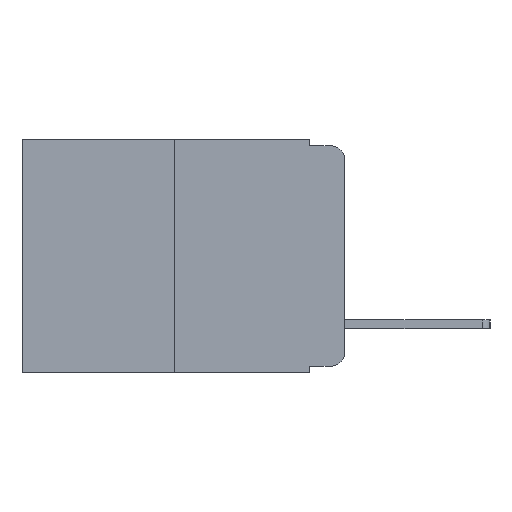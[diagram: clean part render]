
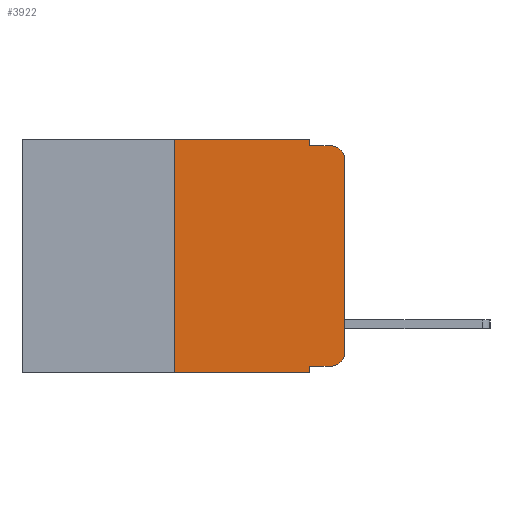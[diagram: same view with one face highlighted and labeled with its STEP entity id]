
A CAD part, left-side view. The second image highlights one B-rep face of the part: STEP entity #3922.
In plain terms, the highlighted planar face has unit normal (-1, 0, 0).
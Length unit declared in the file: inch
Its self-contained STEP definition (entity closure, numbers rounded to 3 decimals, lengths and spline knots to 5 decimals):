
#48 = PLANE ( 'NONE',  #1710 ) ;
#73 = DIRECTION ( 'NONE',  ( 0., 0., -1. ) ) ;
#90 = DIRECTION ( 'NONE',  ( 1., 0., 0. ) ) ;
#201 = DIRECTION ( 'NONE',  ( 0., 0., 1. ) ) ;
#320 = VERTEX_POINT ( 'NONE', #8663 ) ;
#596 = DIRECTION ( 'NONE',  ( 0., 0., -1. ) ) ;
#610 = VECTOR ( 'NONE', #3336, 39.37008 ) ;
#763 = EDGE_CURVE ( 'NONE', #1089, #12890, #6346, .T. ) ;
#775 = AXIS2_PLACEMENT_3D ( 'NONE', #8355, #8340, #7607 ) ;
#857 = CARTESIAN_POINT ( 'NONE',  ( 0., 0.25, 0. ) ) ;
#897 = CARTESIAN_POINT ( 'NONE',  ( 0., 0.25, 0. ) ) ;
#1089 = VERTEX_POINT ( 'NONE', #10288 ) ;
#1657 = EDGE_CURVE ( 'NONE', #2693, #8199, #9478, .T. ) ;
#1710 = AXIS2_PLACEMENT_3D ( 'NONE', #6113, #90, #73 ) ;
#2004 = ORIENTED_EDGE ( 'NONE', *, *, #11874, .T. ) ;
#2117 = CARTESIAN_POINT ( 'NONE',  ( 0., 0.051, 0. ) ) ;
#2319 = CARTESIAN_POINT ( 'NONE',  ( 0., 0., 0. ) ) ;
#2333 = ORIENTED_EDGE ( 'NONE', *, *, #3789, .T. ) ;
#2411 = CARTESIAN_POINT ( 'NONE',  ( 0., 0.051, -0.01 ) ) ;
#2581 = CARTESIAN_POINT ( 'NONE',  ( 0., 0.473, 0. ) ) ;
#2693 = VERTEX_POINT ( 'NONE', #897 ) ;
#2996 = VERTEX_POINT ( 'NONE', #2411 ) ;
#3309 = ORIENTED_EDGE ( 'NONE', *, *, #3371, .T. ) ;
#3336 = DIRECTION ( 'NONE',  ( 0., 0., -1. ) ) ;
#3371 = EDGE_CURVE ( 'NONE', #9353, #320, #12483, .T. ) ;
#3393 = LINE ( 'NONE', #2319, #8781 ) ;
#3564 = DIRECTION ( 'NONE',  ( 0., -1., 0. ) ) ;
#3789 = EDGE_CURVE ( 'NONE', #12726, #10171, #4030, .T. ) ;
#3831 = DIRECTION ( 'NONE',  ( 0., -1., 0. ) ) ;
#3922 = ADVANCED_FACE ( 'NONE', ( #8435 ), #48, .F. ) ;
#4030 = CIRCLE ( 'NONE', #6306, 0.02 ) ;
#4320 = ORIENTED_EDGE ( 'NONE', *, *, #12712, .F. ) ;
#4924 = CARTESIAN_POINT ( 'NONE',  ( 0., 0., -0.03 ) ) ;
#4969 = VECTOR ( 'NONE', #10505, 39.37008 ) ;
#4999 = VERTEX_POINT ( 'NONE', #11763 ) ;
#5079 = VECTOR ( 'NONE', #3831, 39.37008 ) ;
#5171 = VECTOR ( 'NONE', #9174, 39.37008 ) ;
#5239 = EDGE_CURVE ( 'NONE', #4999, #12890, #10244, .T. ) ;
#5328 = CARTESIAN_POINT ( 'NONE',  ( 0., 0.051, -0.343 ) ) ;
#5497 = LINE ( 'NONE', #8148, #5171 ) ;
#5764 = VECTOR ( 'NONE', #596, 39.37008 ) ;
#5983 = CARTESIAN_POINT ( 'NONE',  ( 0., 0.051, 0. ) ) ;
#6113 = CARTESIAN_POINT ( 'NONE',  ( 0., 0.473, 0. ) ) ;
#6256 = CARTESIAN_POINT ( 'NONE',  ( 0., 0.02, -0.01 ) ) ;
#6306 = AXIS2_PLACEMENT_3D ( 'NONE', #8937, #8924, #8656 ) ;
#6346 = LINE ( 'NONE', #2117, #610 ) ;
#6384 = ORIENTED_EDGE ( 'NONE', *, *, #5239, .T. ) ;
#6559 = EDGE_LOOP ( 'NONE', ( #2004, #2333, #11455, #4320, #10643, #8547, #6384, #9543, #7746, #3309 ) ) ;
#7472 = VECTOR ( 'NONE', #12416, 39.37008 ) ;
#7560 = CARTESIAN_POINT ( 'NONE',  ( 0., 0.051, 0. ) ) ;
#7607 = DIRECTION ( 'NONE',  ( 0., 0., -1. ) ) ;
#7746 = ORIENTED_EDGE ( 'NONE', *, *, #12145, .T. ) ;
#7894 = EDGE_CURVE ( 'NONE', #2996, #10171, #5497, .T. ) ;
#8025 = CARTESIAN_POINT ( 'NONE',  ( 0., 0.02, -0.333 ) ) ;
#8148 = CARTESIAN_POINT ( 'NONE',  ( 0., 0.051, -0.01 ) ) ;
#8199 = VERTEX_POINT ( 'NONE', #7560 ) ;
#8340 = DIRECTION ( 'NONE',  ( -1., 0., 0. ) ) ;
#8355 = CARTESIAN_POINT ( 'NONE',  ( 0., 0.02, -0.313 ) ) ;
#8435 = FACE_OUTER_BOUND ( 'NONE', #6559, .T. ) ;
#8547 = ORIENTED_EDGE ( 'NONE', *, *, #8965, .F. ) ;
#8613 = LINE ( 'NONE', #5983, #5764 ) ;
#8656 = DIRECTION ( 'NONE',  ( 0., 0., -1. ) ) ;
#8663 = CARTESIAN_POINT ( 'NONE',  ( 0., 0., -0.313 ) ) ;
#8781 = VECTOR ( 'NONE', #201, 39.37008 ) ;
#8924 = DIRECTION ( 'NONE',  ( -1., 0., 0. ) ) ;
#8937 = CARTESIAN_POINT ( 'NONE',  ( 0., 0.02, -0.03 ) ) ;
#8965 = EDGE_CURVE ( 'NONE', #4999, #2693, #13377, .T. ) ;
#9152 = VECTOR ( 'NONE', #3564, 39.37008 ) ;
#9157 = CARTESIAN_POINT ( 'NONE',  ( 0., 0.051, -0.333 ) ) ;
#9174 = DIRECTION ( 'NONE',  ( 0., -1., 0. ) ) ;
#9353 = VERTEX_POINT ( 'NONE', #8025 ) ;
#9478 = LINE ( 'NONE', #2581, #9152 ) ;
#9543 = ORIENTED_EDGE ( 'NONE', *, *, #763, .F. ) ;
#10171 = VERTEX_POINT ( 'NONE', #6256 ) ;
#10244 = LINE ( 'NONE', #12430, #7472 ) ;
#10288 = CARTESIAN_POINT ( 'NONE',  ( 0., 0.051, -0.333 ) ) ;
#10505 = DIRECTION ( 'NONE',  ( 0., 0., 1. ) ) ;
#10643 = ORIENTED_EDGE ( 'NONE', *, *, #1657, .F. ) ;
#11366 = LINE ( 'NONE', #9157, #5079 ) ;
#11455 = ORIENTED_EDGE ( 'NONE', *, *, #7894, .F. ) ;
#11763 = CARTESIAN_POINT ( 'NONE',  ( 0., 0.25, -0.343 ) ) ;
#11874 = EDGE_CURVE ( 'NONE', #320, #12726, #3393, .T. ) ;
#12145 = EDGE_CURVE ( 'NONE', #1089, #9353, #11366, .T. ) ;
#12416 = DIRECTION ( 'NONE',  ( 0., -1., 0. ) ) ;
#12430 = CARTESIAN_POINT ( 'NONE',  ( 0., 0.473, -0.343 ) ) ;
#12483 = CIRCLE ( 'NONE', #775, 0.02 ) ;
#12712 = EDGE_CURVE ( 'NONE', #8199, #2996, #8613, .T. ) ;
#12726 = VERTEX_POINT ( 'NONE', #4924 ) ;
#12890 = VERTEX_POINT ( 'NONE', #5328 ) ;
#13377 = LINE ( 'NONE', #857, #4969 ) ;
